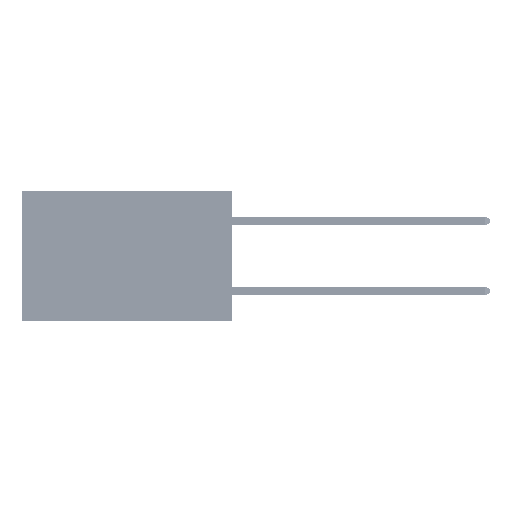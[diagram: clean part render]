
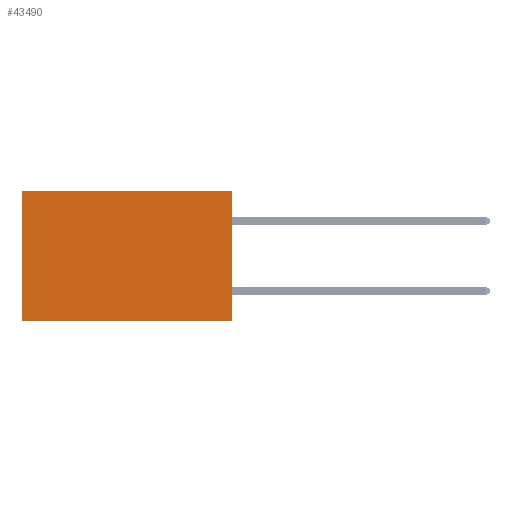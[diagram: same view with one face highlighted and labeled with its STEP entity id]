
A CAD part, left-side view. The second image highlights one B-rep face of the part: STEP entity #43490.
In plain terms, the highlighted planar face has unit normal (-1, 0, 0).
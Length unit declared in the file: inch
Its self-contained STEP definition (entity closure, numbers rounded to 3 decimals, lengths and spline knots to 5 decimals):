
#2918 = DIRECTION ( 'NONE',  ( 0., 0., -1. ) ) ;
#7414 = ORIENTED_EDGE ( 'NONE', *, *, #41082, .F. ) ;
#9553 = CARTESIAN_POINT ( 'NONE',  ( 0.2875, 0., 0. ) ) ;
#10796 = DIRECTION ( 'NONE',  ( 1., 0., 0. ) ) ;
#11060 = CARTESIAN_POINT ( 'NONE',  ( 0.2875, 0.6, -0.37 ) ) ;
#14246 = FACE_OUTER_BOUND ( 'NONE', #36554, .T. ) ;
#15867 = VECTOR ( 'NONE', #39544, 39.37008 ) ;
#17180 = CARTESIAN_POINT ( 'NONE',  ( 0.2875, 0., 0. ) ) ;
#18092 = VECTOR ( 'NONE', #2918, 39.37008 ) ;
#18280 = DIRECTION ( 'NONE',  ( 0., 0., -1. ) ) ;
#19880 = ORIENTED_EDGE ( 'NONE', *, *, #37938, .F. ) ;
#20463 = VERTEX_POINT ( 'NONE', #17180 ) ;
#21347 = ORIENTED_EDGE ( 'NONE', *, *, #24573, .T. ) ;
#21765 = VECTOR ( 'NONE', #40276, 39.37008 ) ;
#22594 = DIRECTION ( 'NONE',  ( 0., 0., -1. ) ) ;
#23083 = LINE ( 'NONE', #38172, #32117 ) ;
#24573 = EDGE_CURVE ( 'NONE', #24732, #38596, #23083, .T. ) ;
#24732 = VERTEX_POINT ( 'NONE', #27103 ) ;
#25726 = CARTESIAN_POINT ( 'NONE',  ( 0.2875, 0., 0. ) ) ;
#27103 = CARTESIAN_POINT ( 'NONE',  ( 0.2875, 0.6, 0. ) ) ;
#29021 = VERTEX_POINT ( 'NONE', #43927 ) ;
#29728 = ORIENTED_EDGE ( 'NONE', *, *, #45304, .T. ) ;
#32117 = VECTOR ( 'NONE', #22594, 39.37008 ) ;
#32216 = CARTESIAN_POINT ( 'NONE',  ( 0.2875, 0., -0.37 ) ) ;
#33847 = LINE ( 'NONE', #32216, #15867 ) ;
#34178 = LINE ( 'NONE', #25726, #18092 ) ;
#36554 = EDGE_LOOP ( 'NONE', ( #21347, #19880, #7414, #29728 ) ) ;
#36886 = CARTESIAN_POINT ( 'NONE',  ( 0.2875, 0., 0. ) ) ;
#37938 = EDGE_CURVE ( 'NONE', #29021, #38596, #33847, .T. ) ;
#38172 = CARTESIAN_POINT ( 'NONE',  ( 0.2875, 0.6, 0. ) ) ;
#38596 = VERTEX_POINT ( 'NONE', #11060 ) ;
#39544 = DIRECTION ( 'NONE',  ( 0., 1., 0. ) ) ;
#40276 = DIRECTION ( 'NONE',  ( 0., 1., 0. ) ) ;
#41082 = EDGE_CURVE ( 'NONE', #20463, #29021, #34178, .T. ) ;
#43283 = LINE ( 'NONE', #9553, #21765 ) ;
#43490 = ADVANCED_FACE ( 'NONE', ( #14246 ), #48364, .F. ) ;
#43927 = CARTESIAN_POINT ( 'NONE',  ( 0.2875, 0., -0.37 ) ) ;
#45304 = EDGE_CURVE ( 'NONE', #20463, #24732, #43283, .T. ) ;
#48364 = PLANE ( 'NONE',  #48799 ) ;
#48799 = AXIS2_PLACEMENT_3D ( 'NONE', #36886, #10796, #18280 ) ;
